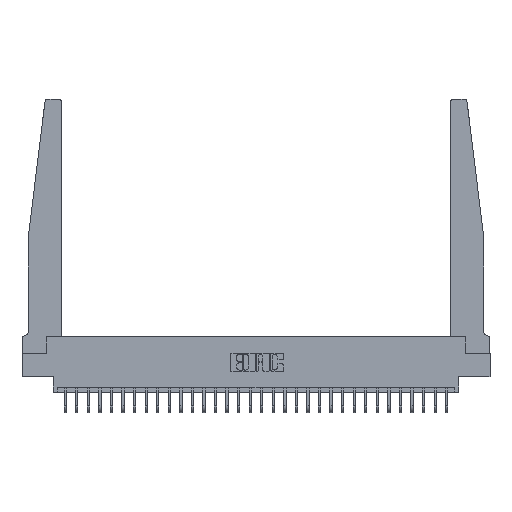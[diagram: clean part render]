
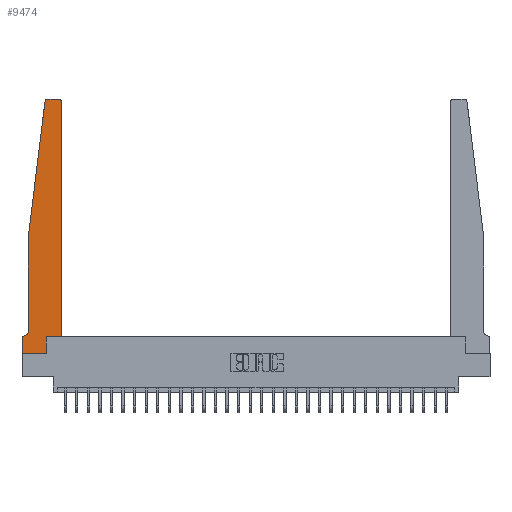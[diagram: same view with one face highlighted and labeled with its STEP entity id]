
A CAD part, top view. The second image highlights one B-rep face of the part: STEP entity #9474.
In plain terms, the highlighted planar face has unit normal (0, 0, 1).
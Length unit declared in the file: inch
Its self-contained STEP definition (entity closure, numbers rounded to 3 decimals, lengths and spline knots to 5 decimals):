
#233 = CARTESIAN_POINT ( 'NONE',  ( 0.065, 0.2375, 0.37 ) ) ;
#334 = CARTESIAN_POINT ( 'NONE',  ( 0.25, 2.75, 0.37 ) ) ;
#698 = AXIS2_PLACEMENT_3D ( 'NONE', #14546, #12530, #803 ) ;
#803 = DIRECTION ( 'NONE',  ( -1., 0., 0. ) ) ;
#829 = EDGE_CURVE ( 'NONE', #19472, #2633, #5555, .T. ) ;
#1214 = VECTOR ( 'NONE', #5824, 39.37008 ) ;
#1306 = CARTESIAN_POINT ( 'NONE',  ( 0.425, 0.18, 0.37 ) ) ;
#1307 = AXIS2_PLACEMENT_3D ( 'NONE', #16108, #4628, #16906 ) ;
#1423 = VECTOR ( 'NONE', #23205, 39.37008 ) ;
#2256 = CARTESIAN_POINT ( 'NONE',  ( 0.2605, 0., 0.37 ) ) ;
#2588 = EDGE_CURVE ( 'NONE', #4914, #19699, #10598, .T. ) ;
#2633 = VERTEX_POINT ( 'NONE', #7050 ) ;
#2788 = EDGE_CURVE ( 'NONE', #7664, #23280, #26886, .T. ) ;
#3637 = VECTOR ( 'NONE', #8344, 39.37008 ) ;
#4036 = EDGE_CURVE ( 'NONE', #19699, #29823, #16608, .T. ) ;
#4322 = VECTOR ( 'NONE', #25476, 39.37008 ) ;
#4595 = AXIS2_PLACEMENT_3D ( 'NONE', #5299, #21455, #10337 ) ;
#4628 = DIRECTION ( 'NONE',  ( 0., 0., 1. ) ) ;
#4805 = VERTEX_POINT ( 'NONE', #233 ) ;
#4914 = VERTEX_POINT ( 'NONE', #23937 ) ;
#4955 = EDGE_CURVE ( 'NONE', #23280, #23550, #12969, .T. ) ;
#5299 = CARTESIAN_POINT ( 'NONE',  ( 0.27653, 2.72, 0.37 ) ) ;
#5555 = LINE ( 'NONE', #1306, #29438 ) ;
#5824 = DIRECTION ( 'NONE',  ( 0., 1., 0. ) ) ;
#6115 = ORIENTED_EDGE ( 'NONE', *, *, #14141, .T. ) ;
#6574 = VECTOR ( 'NONE', #7271, 39.37008 ) ;
#6758 = FACE_OUTER_BOUND ( 'NONE', #10787, .T. ) ;
#7050 = CARTESIAN_POINT ( 'NONE',  ( 0.425, 0.18, 0.37 ) ) ;
#7271 = DIRECTION ( 'NONE',  ( 0., -1., 0. ) ) ;
#7522 = VECTOR ( 'NONE', #10163, 39.37008 ) ;
#7664 = VERTEX_POINT ( 'NONE', #11892 ) ;
#7777 = CIRCLE ( 'NONE', #698, 0.05 ) ;
#7859 = EDGE_CURVE ( 'NONE', #29823, #19472, #13890, .T. ) ;
#8142 = ORIENTED_EDGE ( 'NONE', *, *, #2788, .T. ) ;
#8344 = DIRECTION ( 'NONE',  ( 1., 0., 0. ) ) ;
#8439 = EDGE_CURVE ( 'NONE', #23550, #14074, #15670, .T. ) ;
#8890 = DIRECTION ( 'NONE',  ( -1., 0., 0. ) ) ;
#8994 = LINE ( 'NONE', #16006, #4322 ) ;
#9350 = CARTESIAN_POINT ( 'NONE',  ( 0.015, 0.1875, 0.37 ) ) ;
#9474 = ADVANCED_FACE ( 'NONE', ( #6758 ), #25575, .T. ) ;
#9762 = CARTESIAN_POINT ( 'NONE',  ( 0.24675, 2.72367, 0.37 ) ) ;
#9973 = CARTESIAN_POINT ( 'NONE',  ( 0.2605, 0.18, 0.37 ) ) ;
#10106 = CARTESIAN_POINT ( 'NONE',  ( 0.395, 2.75, 0.37 ) ) ;
#10163 = DIRECTION ( 'NONE',  ( 0., 1., 0. ) ) ;
#10337 = DIRECTION ( 'NONE',  ( 1., 0., 0. ) ) ;
#10593 = CARTESIAN_POINT ( 'NONE',  ( 0., 0., 0.37 ) ) ;
#10598 = LINE ( 'NONE', #28625, #29040 ) ;
#10700 = ORIENTED_EDGE ( 'NONE', *, *, #12608, .T. ) ;
#10787 = EDGE_LOOP ( 'NONE', ( #27395, #19920, #27621, #10700, #28126, #18814, #19365, #10974, #14468, #19836, #6115, #8142 ) ) ;
#10974 = ORIENTED_EDGE ( 'NONE', *, *, #4036, .T. ) ;
#11196 = LINE ( 'NONE', #14689, #7522 ) ;
#11892 = CARTESIAN_POINT ( 'NONE',  ( 0.425, 2.72, 0.37 ) ) ;
#11972 = VECTOR ( 'NONE', #8890, 39.37008 ) ;
#12196 = VERTEX_POINT ( 'NONE', #26842 ) ;
#12530 = DIRECTION ( 'NONE',  ( 0., 0., -1. ) ) ;
#12608 = EDGE_CURVE ( 'NONE', #12196, #4805, #16653, .T. ) ;
#12961 = AXIS2_PLACEMENT_3D ( 'NONE', #29254, #15367, #17795 ) ;
#12969 = LINE ( 'NONE', #334, #1423 ) ;
#13890 = LINE ( 'NONE', #24452, #1214 ) ;
#14074 = VERTEX_POINT ( 'NONE', #9762 ) ;
#14141 = EDGE_CURVE ( 'NONE', #2633, #7664, #11196, .T. ) ;
#14468 = ORIENTED_EDGE ( 'NONE', *, *, #7859, .T. ) ;
#14546 = CARTESIAN_POINT ( 'NONE',  ( 0.015, 0.2375, 0.37 ) ) ;
#14689 = CARTESIAN_POINT ( 'NONE',  ( 0.425, 0.18, 0.37 ) ) ;
#15367 = DIRECTION ( 'NONE',  ( 0., 0., 1. ) ) ;
#15670 = CIRCLE ( 'NONE', #4595, 0.03 ) ;
#16006 = CARTESIAN_POINT ( 'NONE',  ( 0.065, 1.25, 0.37 ) ) ;
#16108 = CARTESIAN_POINT ( 'NONE',  ( 0., 0.1875, 0.37 ) ) ;
#16608 = LINE ( 'NONE', #10593, #3637 ) ;
#16638 = LINE ( 'NONE', #24712, #11972 ) ;
#16653 = LINE ( 'NONE', #21118, #6574 ) ;
#16906 = DIRECTION ( 'NONE',  ( 1., 0., 0. ) ) ;
#16959 = VERTEX_POINT ( 'NONE', #9350 ) ;
#16971 = EDGE_CURVE ( 'NONE', #14074, #12196, #8994, .T. ) ;
#17795 = DIRECTION ( 'NONE',  ( 1., 0., 0. ) ) ;
#18154 = DIRECTION ( 'NONE',  ( 1., 0., 0. ) ) ;
#18814 = ORIENTED_EDGE ( 'NONE', *, *, #21883, .T. ) ;
#18979 = EDGE_CURVE ( 'NONE', #4805, #16959, #7777, .T. ) ;
#19365 = ORIENTED_EDGE ( 'NONE', *, *, #2588, .T. ) ;
#19472 = VERTEX_POINT ( 'NONE', #9973 ) ;
#19699 = VERTEX_POINT ( 'NONE', #29188 ) ;
#19786 = CARTESIAN_POINT ( 'NONE',  ( 0.27653, 2.75, 0.37 ) ) ;
#19836 = ORIENTED_EDGE ( 'NONE', *, *, #829, .T. ) ;
#19920 = ORIENTED_EDGE ( 'NONE', *, *, #8439, .T. ) ;
#21118 = CARTESIAN_POINT ( 'NONE',  ( 0.065, 1.25, 0.37 ) ) ;
#21455 = DIRECTION ( 'NONE',  ( 0., 0., 1. ) ) ;
#21883 = EDGE_CURVE ( 'NONE', #16959, #4914, #16638, .T. ) ;
#23205 = DIRECTION ( 'NONE',  ( -1., 0., 0. ) ) ;
#23280 = VERTEX_POINT ( 'NONE', #10106 ) ;
#23550 = VERTEX_POINT ( 'NONE', #19786 ) ;
#23937 = CARTESIAN_POINT ( 'NONE',  ( 0., 0.1875, 0.37 ) ) ;
#24452 = CARTESIAN_POINT ( 'NONE',  ( 0.2605, 0.18, 0.37 ) ) ;
#24712 = CARTESIAN_POINT ( 'NONE',  ( 0.065, 0.1875, 0.37 ) ) ;
#25476 = DIRECTION ( 'NONE',  ( -0.122, -0.992, 0. ) ) ;
#25575 = PLANE ( 'NONE',  #1307 ) ;
#26842 = CARTESIAN_POINT ( 'NONE',  ( 0.065, 1.25, 0.37 ) ) ;
#26886 = CIRCLE ( 'NONE', #12961, 0.03 ) ;
#26914 = DIRECTION ( 'NONE',  ( 0., -1., 0. ) ) ;
#27395 = ORIENTED_EDGE ( 'NONE', *, *, #4955, .T. ) ;
#27621 = ORIENTED_EDGE ( 'NONE', *, *, #16971, .T. ) ;
#28126 = ORIENTED_EDGE ( 'NONE', *, *, #18979, .T. ) ;
#28625 = CARTESIAN_POINT ( 'NONE',  ( 0., 0., 0.37 ) ) ;
#29040 = VECTOR ( 'NONE', #26914, 39.37008 ) ;
#29188 = CARTESIAN_POINT ( 'NONE',  ( 0., 0., 0.37 ) ) ;
#29254 = CARTESIAN_POINT ( 'NONE',  ( 0.395, 2.72, 0.37 ) ) ;
#29438 = VECTOR ( 'NONE', #18154, 39.37008 ) ;
#29823 = VERTEX_POINT ( 'NONE', #2256 ) ;
